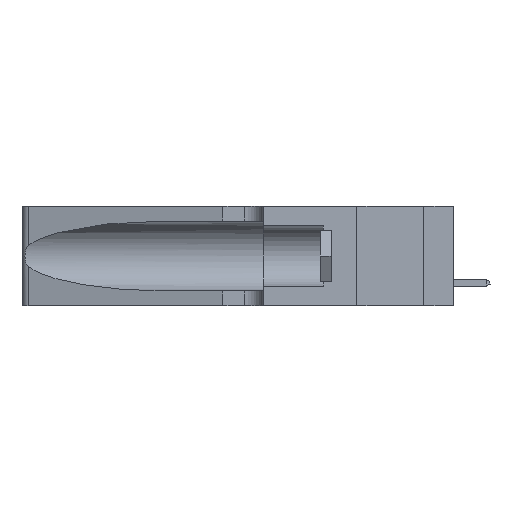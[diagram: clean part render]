
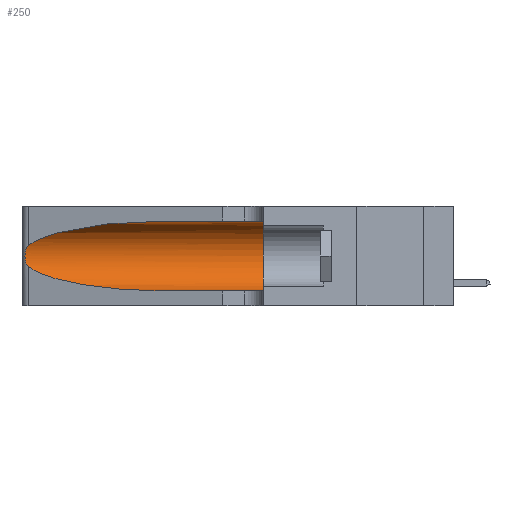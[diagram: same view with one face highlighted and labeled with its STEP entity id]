
A CAD part, left-side view. The second image highlights one B-rep face of the part: STEP entity #250.
In plain terms, the highlighted cylindrical face has radius 3.308 mm (diameter 6.617 mm), a partial arc.
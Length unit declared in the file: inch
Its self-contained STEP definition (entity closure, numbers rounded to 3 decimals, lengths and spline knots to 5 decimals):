
#250 = ADVANCED_FACE ( 'NONE', ( #9696 ), #25543, .F. ) ;
#454 = EDGE_CURVE ( 'NONE', #20130, #5412, #11049, .T. ) ;
#609 = CARTESIAN_POINT ( 'NONE',  ( 0.1305, 0.72297, 0.05475 ) ) ;
#865 = CARTESIAN_POINT ( 'NONE',  ( 0.25854, 1.2359, 0.20912 ) ) ;
#981 = CARTESIAN_POINT ( 'NONE',  ( 0.25555, 1.22993, 0.14849 ) ) ;
#1940 = CARTESIAN_POINT ( 'NONE',  ( 0.1305, 0.72297, 0.05475 ) ) ;
#2172 = CARTESIAN_POINT ( 'NONE',  ( 0.1305, 1.61858, 0.185 ) ) ;
#3123 = VERTEX_POINT ( 'NONE', #13155 ) ;
#3322 = CARTESIAN_POINT ( 'NONE',  ( 0.25487, 1.22718, 0.14631 ) ) ;
#3418 = CARTESIAN_POINT ( 'NONE',  ( 0.25555, 1.22994, 0.2215 ) ) ;
#3536 = CARTESIAN_POINT ( 'NONE',  ( 0.26075, 1.23896, 0.19203 ) ) ;
#3650 = CARTESIAN_POINT ( 'NONE',  ( 0.25787, 1.23484, 0.2124 ) ) ;
#4032 = CARTESIAN_POINT ( 'NONE',  ( 0.1305, 0.72297, 0.31525 ) ) ;
#4229 = VERTEX_POINT ( 'NONE', #19059 ) ;
#4381 = ORIENTED_EDGE ( 'NONE', *, *, #19094, .F. ) ;
#4875 = CARTESIAN_POINT ( 'NONE',  ( 0.1305, 1.61858, 0.31525 ) ) ;
#5412 = VERTEX_POINT ( 'NONE', #1940 ) ;
#5697 = CARTESIAN_POINT ( 'NONE',  ( 0.1305, 1.61858, 0.05475 ) ) ;
#5870 = CARTESIAN_POINT ( 'NONE',  ( 0.25487, 1.22718, 0.14631 ) ) ;
#6172 = EDGE_CURVE ( 'NONE', #28967, #17515, #10030, .T. ) ;
#6266 = CARTESIAN_POINT ( 'NONE',  ( 0.26017, 1.23833, 0.17102 ) ) ;
#6354 = AXIS2_PLACEMENT_3D ( 'NONE', #24773, #19672, #25118 ) ;
#6606 = CARTESIAN_POINT ( 'NONE',  ( 0.25487, 1.22718, 0.22369 ) ) ;
#7215 = CIRCLE ( 'NONE', #6354, 0.13025 ) ;
#8663 = CARTESIAN_POINT ( 'NONE',  ( 0.18966, 0.96281, 0.05475 ) ) ;
#8931 = CARTESIAN_POINT ( 'NONE',  ( 0.25639, 1.23186, 0.15144 ) ) ;
#9696 = FACE_OUTER_BOUND ( 'NONE', #27639, .T. ) ;
#9881 = VECTOR ( 'NONE', #29800, 39.37008 ) ;
#10030 = LINE ( 'NONE', #4875, #11268 ) ;
#10357 = DIRECTION ( 'NONE',  ( 0., -1., 0. ) ) ;
#11003 = ORIENTED_EDGE ( 'NONE', *, *, #25398, .T. ) ;
#11049 =( BOUNDED_CURVE ( )  B_SPLINE_CURVE ( 3, ( #5870, #32537, #8663, #609 ),
 .UNSPECIFIED., .F., .F. ) 
 B_SPLINE_CURVE_WITH_KNOTS ( ( 4, 4 ),
 ( 3.44316, 4.71239 ),
 .UNSPECIFIED. ) 
 CURVE ( )  GEOMETRIC_REPRESENTATION_ITEM ( )  RATIONAL_B_SPLINE_CURVE ( ( 1., 0.87, 0.87, 1. ) ) 
 REPRESENTATION_ITEM ( '' )  );
#11268 = VECTOR ( 'NONE', #10357, 39.37008 ) ;
#11503 = CARTESIAN_POINT ( 'NONE',  ( 0.2373, 1.15595, 0.28018 ) ) ;
#12820 = CARTESIAN_POINT ( 'NONE',  ( 0.1305, 0.35, 0.31525 ) ) ;
#13155 = CARTESIAN_POINT ( 'NONE',  ( 0.25487, 1.22718, 0.22369 ) ) ;
#13213 = DIRECTION ( 'NONE',  ( 0., 0., -1. ) ) ;
#13565 = EDGE_CURVE ( 'NONE', #5412, #4229, #20338, .T. ) ;
#16656 = B_SPLINE_CURVE_WITH_KNOTS ( 'NONE', 3,
 ( #6606, #3418, #16871, #3650, #865, #19519, #3536, #22195, #6266, #16986, #24864, #8931, #981, #30689 ),
 .UNSPECIFIED., .F., .F.,
 ( 4, 2, 2, 2, 2, 2, 4 ),
 ( 0., 0.00027, 0.00053, 0.00107, 0.0016, 0.00187, 0.00214 ),
 .UNSPECIFIED. ) ;
#16798 = CARTESIAN_POINT ( 'NONE',  ( 0.18966, 0.96281, 0.31525 ) ) ;
#16871 = CARTESIAN_POINT ( 'NONE',  ( 0.25639, 1.23184, 0.21858 ) ) ;
#16986 = CARTESIAN_POINT ( 'NONE',  ( 0.25856, 1.23593, 0.16098 ) ) ;
#17515 = VERTEX_POINT ( 'NONE', #12820 ) ;
#19059 = CARTESIAN_POINT ( 'NONE',  ( 0.1305, 0.35, 0.05475 ) ) ;
#19094 = EDGE_CURVE ( 'NONE', #17515, #4229, #7215, .T. ) ;
#19519 = CARTESIAN_POINT ( 'NONE',  ( 0.26018, 1.23835, 0.19895 ) ) ;
#19672 = DIRECTION ( 'NONE',  ( 0., 1., 0. ) ) ;
#19788 = ORIENTED_EDGE ( 'NONE', *, *, #28751, .T. ) ;
#20130 = VERTEX_POINT ( 'NONE', #3322 ) ;
#20314 =( BOUNDED_CURVE ( )  B_SPLINE_CURVE ( 3, ( #32728, #16798, #11503, #30143 ),
 .UNSPECIFIED., .F., .F. ) 
 B_SPLINE_CURVE_WITH_KNOTS ( ( 4, 4 ),
 ( 1.5708, 2.84003 ),
 .UNSPECIFIED. ) 
 CURVE ( )  GEOMETRIC_REPRESENTATION_ITEM ( )  RATIONAL_B_SPLINE_CURVE ( ( 1., 0.87, 0.87, 1. ) ) 
 REPRESENTATION_ITEM ( '' )  );
#20338 = LINE ( 'NONE', #5697, #9881 ) ;
#20501 = DIRECTION ( 'NONE',  ( 0., -1., 0. ) ) ;
#20503 = AXIS2_PLACEMENT_3D ( 'NONE', #2172, #20501, #13213 ) ;
#22195 = CARTESIAN_POINT ( 'NONE',  ( 0.26075, 1.23896, 0.178 ) ) ;
#24773 = CARTESIAN_POINT ( 'NONE',  ( 0.1305, 0.35, 0.185 ) ) ;
#24864 = CARTESIAN_POINT ( 'NONE',  ( 0.25789, 1.23486, 0.15765 ) ) ;
#25118 = DIRECTION ( 'NONE',  ( 0., 0., 1. ) ) ;
#25398 = EDGE_CURVE ( 'NONE', #3123, #20130, #16656, .T. ) ;
#25543 = CYLINDRICAL_SURFACE ( 'NONE', #20503, 0.13025 ) ;
#27639 = EDGE_LOOP ( 'NONE', ( #19788, #11003, #33539, #27993, #4381, #33983 ) ) ;
#27993 = ORIENTED_EDGE ( 'NONE', *, *, #13565, .T. ) ;
#28751 = EDGE_CURVE ( 'NONE', #28967, #3123, #20314, .T. ) ;
#28967 = VERTEX_POINT ( 'NONE', #4032 ) ;
#29800 = DIRECTION ( 'NONE',  ( 0., -1., 0. ) ) ;
#30143 = CARTESIAN_POINT ( 'NONE',  ( 0.25487, 1.22718, 0.22369 ) ) ;
#30689 = CARTESIAN_POINT ( 'NONE',  ( 0.25487, 1.22718, 0.14631 ) ) ;
#32537 = CARTESIAN_POINT ( 'NONE',  ( 0.2373, 1.15595, 0.08982 ) ) ;
#32728 = CARTESIAN_POINT ( 'NONE',  ( 0.1305, 0.72297, 0.31525 ) ) ;
#33539 = ORIENTED_EDGE ( 'NONE', *, *, #454, .T. ) ;
#33983 = ORIENTED_EDGE ( 'NONE', *, *, #6172, .F. ) ;
